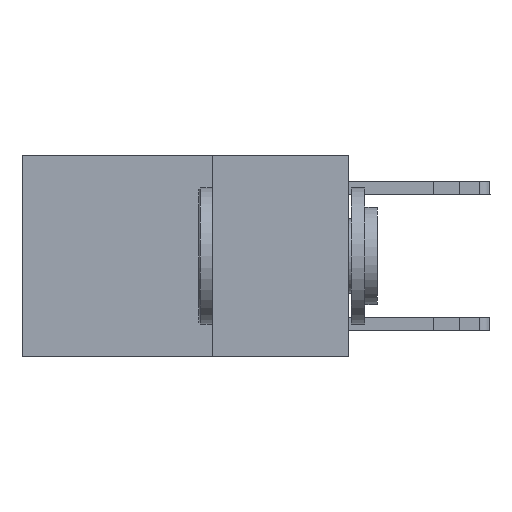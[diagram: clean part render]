
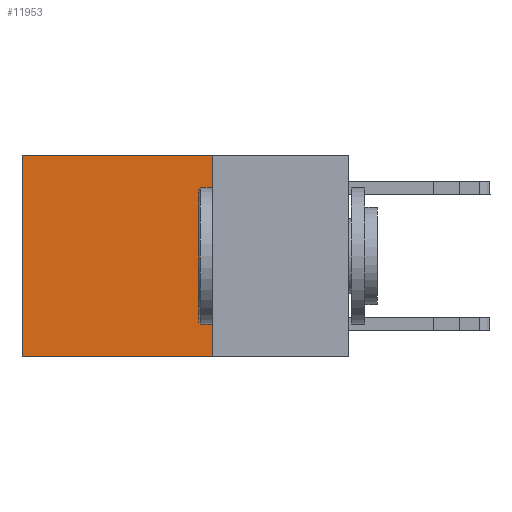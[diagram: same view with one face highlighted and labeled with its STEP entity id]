
A CAD part, left-side view. The second image highlights one B-rep face of the part: STEP entity #11953.
In plain terms, the highlighted planar face has unit normal (-1, 0, 0).
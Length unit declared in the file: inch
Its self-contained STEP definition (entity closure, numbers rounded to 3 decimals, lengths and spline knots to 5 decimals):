
#217 = LINE ( 'NONE', #3498, #1597 ) ;
#589 = VERTEX_POINT ( 'NONE', #18198 ) ;
#954 = CARTESIAN_POINT ( 'NONE',  ( 0.2625, 0.25, -0.37 ) ) ;
#1151 = CARTESIAN_POINT ( 'NONE',  ( 0.2625, 0.25, -0.37 ) ) ;
#1316 = EDGE_CURVE ( 'NONE', #9332, #589, #18096, .T. ) ;
#1380 = DIRECTION ( 'NONE',  ( 0., 1., 0. ) ) ;
#1597 = VECTOR ( 'NONE', #6820, 39.37008 ) ;
#3071 = EDGE_LOOP ( 'NONE', ( #19155, #9105, #21674, #10628 ) ) ;
#3385 = CARTESIAN_POINT ( 'NONE',  ( 0.2625, 0.25, 0. ) ) ;
#3498 = CARTESIAN_POINT ( 'NONE',  ( 0.2625, 0.25, 0. ) ) ;
#3793 = EDGE_CURVE ( 'NONE', #11875, #6743, #16241, .T. ) ;
#4684 = FACE_OUTER_BOUND ( 'NONE', #3071, .T. ) ;
#6445 = DIRECTION ( 'NONE',  ( 1., 0., 0. ) ) ;
#6743 = VERTEX_POINT ( 'NONE', #18965 ) ;
#6820 = DIRECTION ( 'NONE',  ( 0., 0., -1. ) ) ;
#8396 = EDGE_CURVE ( 'NONE', #589, #6743, #12891, .T. ) ;
#8953 = VECTOR ( 'NONE', #15059, 39.37008 ) ;
#9105 = ORIENTED_EDGE ( 'NONE', *, *, #3793, .F. ) ;
#9323 = DIRECTION ( 'NONE',  ( 0., 1., 0. ) ) ;
#9332 = VERTEX_POINT ( 'NONE', #3385 ) ;
#9761 = CARTESIAN_POINT ( 'NONE',  ( 0.2625, 0.25, 0. ) ) ;
#10628 = ORIENTED_EDGE ( 'NONE', *, *, #1316, .T. ) ;
#11875 = VERTEX_POINT ( 'NONE', #954 ) ;
#11953 = ADVANCED_FACE ( 'NONE', ( #4684 ), #14957, .F. ) ;
#12891 = LINE ( 'NONE', #12990, #8953 ) ;
#12990 = CARTESIAN_POINT ( 'NONE',  ( 0.2625, 0.6, 0. ) ) ;
#13148 = VECTOR ( 'NONE', #1380, 39.37008 ) ;
#13536 = VECTOR ( 'NONE', #9323, 39.37008 ) ;
#14957 = PLANE ( 'NONE',  #18190 ) ;
#15059 = DIRECTION ( 'NONE',  ( 0., 0., -1. ) ) ;
#16241 = LINE ( 'NONE', #1151, #13536 ) ;
#18096 = LINE ( 'NONE', #9761, #13148 ) ;
#18190 = AXIS2_PLACEMENT_3D ( 'NONE', #21492, #6445, #19739 ) ;
#18198 = CARTESIAN_POINT ( 'NONE',  ( 0.2625, 0.6, 0. ) ) ;
#18965 = CARTESIAN_POINT ( 'NONE',  ( 0.2625, 0.6, -0.37 ) ) ;
#19155 = ORIENTED_EDGE ( 'NONE', *, *, #8396, .T. ) ;
#19739 = DIRECTION ( 'NONE',  ( 0., 0., -1. ) ) ;
#19775 = EDGE_CURVE ( 'NONE', #9332, #11875, #217, .T. ) ;
#21492 = CARTESIAN_POINT ( 'NONE',  ( 0.2625, 0.25, 0. ) ) ;
#21674 = ORIENTED_EDGE ( 'NONE', *, *, #19775, .F. ) ;
